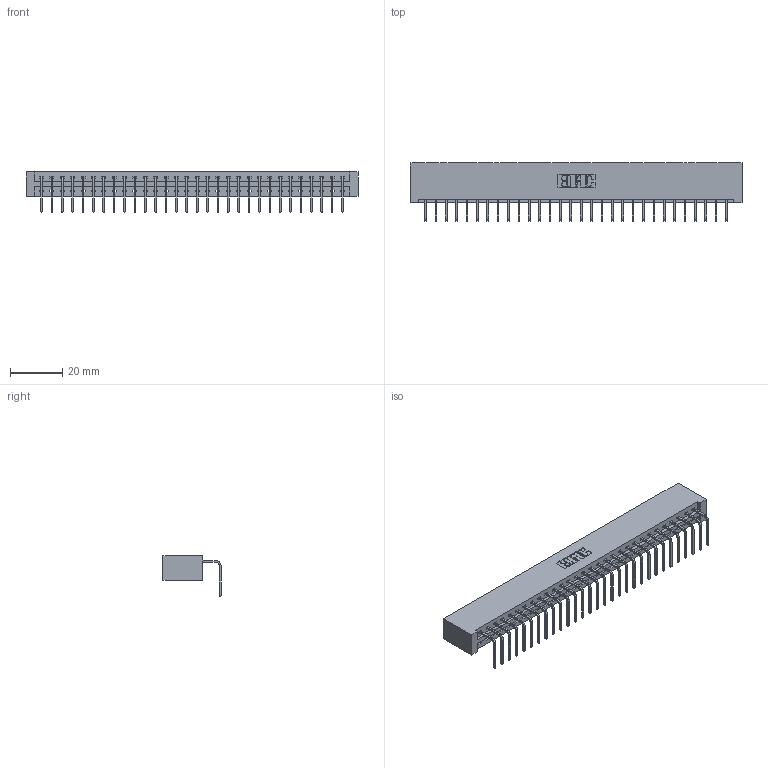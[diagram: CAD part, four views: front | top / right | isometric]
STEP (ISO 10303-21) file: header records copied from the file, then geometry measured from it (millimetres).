
FILE_DESCRIPTION (( 'STEP AP203' ), '1' );
FILE_NAME ('387-030-558-101.STEP', '2019-10-07T19:27:08', ( '' ), ( '' ), 'SwSTEP 2.0', 'SolidWorks 2016', '' );
FILE_SCHEMA (( 'CONFIG_CONTROL_DESIGN' ));
Length unit declared in the file: inch
Products named in the file (3): 337 Part_No Mounting Lugs; 345-292-001_558 Tail - 2; 387-030-558-101
Assembly tree (31 placements, depth 2):
  387-030-558-101
    337 Part_No Mounting Lugs
    345-292-001_558 Tail - 2  x30
Bounding box: 126.75 x 22.17 x 15.37 mm (x, y, z)
Volume: 13861.6 mm3; surface area: 14852.8 mm2
Topology: 31 solids, 31 shells, 2026 faces, 6107 edges, 4030 vertices
Faces by surface type: plane 1506, cylinder 520
Entity records: 23659 total; most frequent: CARTESIAN_POINT 4128, ORIENTED_EDGE 4094, DIRECTION 3491, EDGE_CURVE 2047, LINE 1927, VECTOR 1927, VERTEX_POINT 1362, AXIS2_PLACEMENT_3D 782
